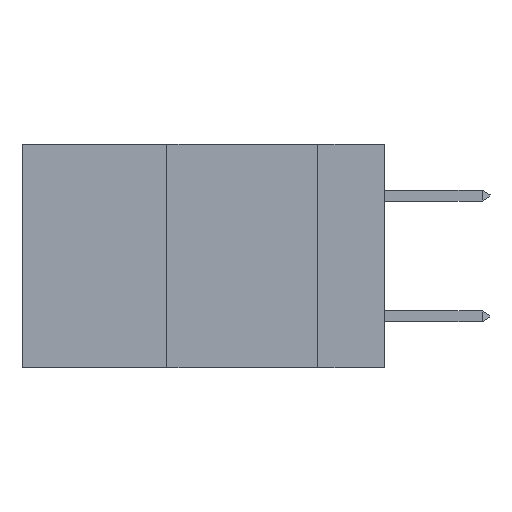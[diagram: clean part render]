
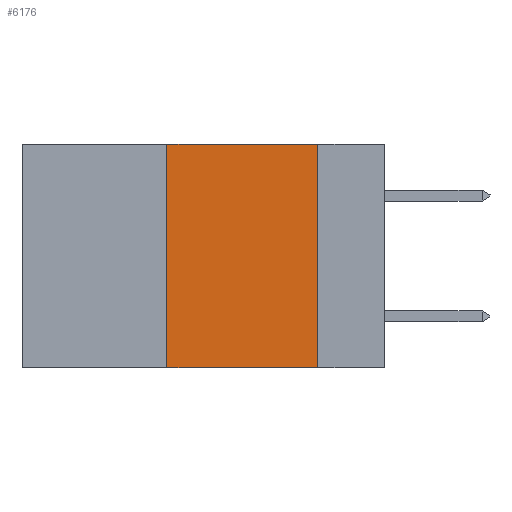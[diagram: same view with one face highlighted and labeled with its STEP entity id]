
A CAD part, left-side view. The second image highlights one B-rep face of the part: STEP entity #6176.
In plain terms, the highlighted planar face has unit normal (-1, 0, 0).
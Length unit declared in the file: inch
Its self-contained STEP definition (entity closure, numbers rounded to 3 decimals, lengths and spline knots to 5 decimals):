
#1091 = ORIENTED_EDGE ( 'NONE', *, *, #15679, .T. ) ;
#1158 = CARTESIAN_POINT ( 'NONE',  ( 0., 0.36, -0.37 ) ) ;
#1590 = VERTEX_POINT ( 'NONE', #15367 ) ;
#1643 = EDGE_CURVE ( 'NONE', #9462, #3942, #12441, .T. ) ;
#2525 = VECTOR ( 'NONE', #15012, 39.37008 ) ;
#3073 = DIRECTION ( 'NONE',  ( 0., -1., 0. ) ) ;
#3177 = ORIENTED_EDGE ( 'NONE', *, *, #1643, .F. ) ;
#3460 = DIRECTION ( 'NONE',  ( 0., 0., 1. ) ) ;
#3898 = CARTESIAN_POINT ( 'NONE',  ( 0., 0.11, -0.37 ) ) ;
#3899 = VERTEX_POINT ( 'NONE', #1158 ) ;
#3942 = VERTEX_POINT ( 'NONE', #3898 ) ;
#4072 = CARTESIAN_POINT ( 'NONE',  ( 0., 0.6, 0. ) ) ;
#4170 = DIRECTION ( 'NONE',  ( 1., 0., 0. ) ) ;
#4503 = ORIENTED_EDGE ( 'NONE', *, *, #15918, .F. ) ;
#4808 = LINE ( 'NONE', #10579, #16954 ) ;
#5315 = PLANE ( 'NONE',  #16479 ) ;
#5504 = DIRECTION ( 'NONE',  ( 0., 0., -1. ) ) ;
#5937 = CARTESIAN_POINT ( 'NONE',  ( 0., 0.6, 0. ) ) ;
#6176 = ADVANCED_FACE ( 'NONE', ( #8351 ), #5315, .F. ) ;
#7940 = EDGE_LOOP ( 'NONE', ( #3177, #8604, #4503, #1091 ) ) ;
#8351 = FACE_OUTER_BOUND ( 'NONE', #7940, .T. ) ;
#8519 = VECTOR ( 'NONE', #17071, 39.37008 ) ;
#8604 = ORIENTED_EDGE ( 'NONE', *, *, #12710, .F. ) ;
#9462 = VERTEX_POINT ( 'NONE', #15381 ) ;
#10579 = CARTESIAN_POINT ( 'NONE',  ( 0., 0.36, 0. ) ) ;
#10908 = VECTOR ( 'NONE', #3073, 39.37008 ) ;
#12441 = LINE ( 'NONE', #16413, #2525 ) ;
#12710 = EDGE_CURVE ( 'NONE', #1590, #9462, #13281, .T. ) ;
#13281 = LINE ( 'NONE', #5937, #10908 ) ;
#15012 = DIRECTION ( 'NONE',  ( 0., 0., -1. ) ) ;
#15367 = CARTESIAN_POINT ( 'NONE',  ( 0., 0.36, 0. ) ) ;
#15381 = CARTESIAN_POINT ( 'NONE',  ( 0., 0.11, 0. ) ) ;
#15679 = EDGE_CURVE ( 'NONE', #3899, #3942, #18319, .T. ) ;
#15918 = EDGE_CURVE ( 'NONE', #3899, #1590, #4808, .T. ) ;
#16413 = CARTESIAN_POINT ( 'NONE',  ( 0., 0.11, 0. ) ) ;
#16479 = AXIS2_PLACEMENT_3D ( 'NONE', #4072, #4170, #5504 ) ;
#16889 = CARTESIAN_POINT ( 'NONE',  ( 0., 0.6, -0.37 ) ) ;
#16954 = VECTOR ( 'NONE', #3460, 39.37008 ) ;
#17071 = DIRECTION ( 'NONE',  ( 0., -1., 0. ) ) ;
#18319 = LINE ( 'NONE', #16889, #8519 ) ;
